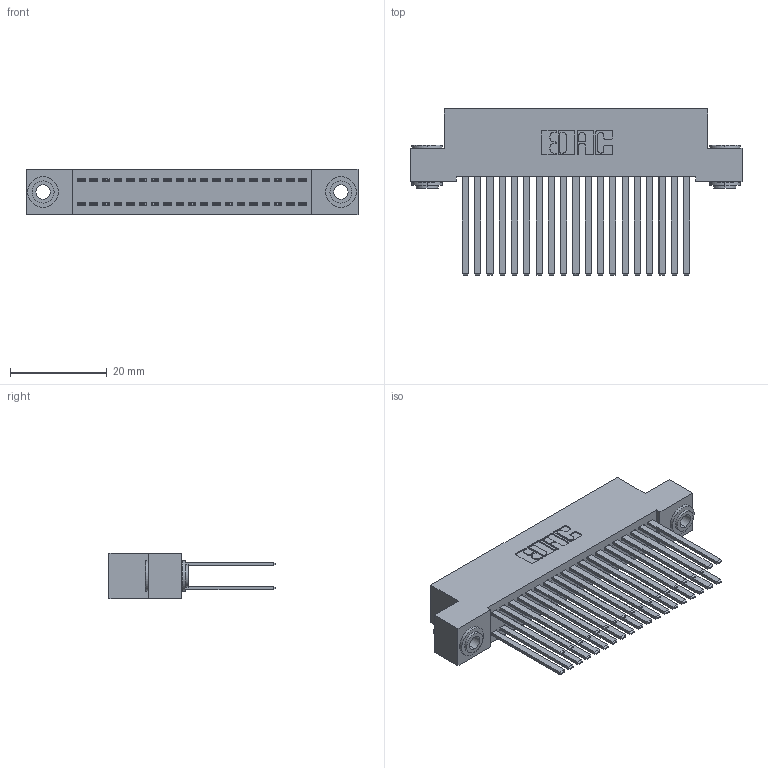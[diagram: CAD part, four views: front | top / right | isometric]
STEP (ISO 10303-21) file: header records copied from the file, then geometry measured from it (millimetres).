
FILE_DESCRIPTION (( 'STEP AP203' ), '1' );
FILE_NAME ('342-038-544-203.STEP', '2018-08-11T22:35:39', ( '' ), ( '' ), 'SwSTEP 2.0', 'SolidWorks 2016', '' );
FILE_SCHEMA (( 'CONFIG_CONTROL_DESIGN' ));
Length unit declared in the file: inch
Products named in the file (4): 342-038-544-203; 342 Part_.156 TH; 345-292-001_345-293-144; 342-250-002_345-250-002-102
Assembly tree (41 placements, depth 2):
  342-038-544-203
    342 Part_.156 TH
    345-292-001_345-293-144  x38
    342-250-002_345-250-002-102  x2
Bounding box: 68.58 x 34.3 x 9.4 mm (x, y, z)
Volume: 6608.5 mm3; surface area: 11879.6 mm2
Topology: 41 solids, 41 shells, 1896 faces, 5581 edges, 3666 vertices
Faces by surface type: plane 1292, cylinder 596, cone 8
Entity records: 15532 total; most frequent: CARTESIAN_POINT 2573, ORIENTED_EDGE 2502, DIRECTION 2269, EDGE_CURVE 1251, VECTOR 1103, LINE 1103, VERTEX_POINT 830, AXIS2_PLACEMENT_3D 583
